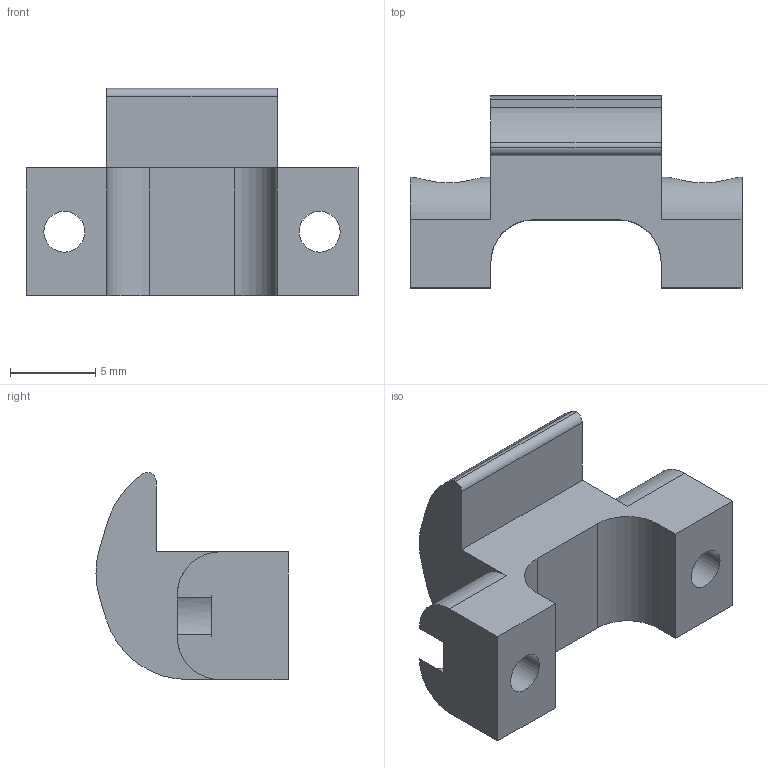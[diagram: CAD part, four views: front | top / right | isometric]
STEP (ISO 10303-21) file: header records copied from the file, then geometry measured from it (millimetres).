
FILE_DESCRIPTION (( 'STEP AP203' ), '1' );
FILE_NAME ('Trigger_Guide.STEP', '2013-11-14T05:08:26', ( '' ), ( '' ), 'SwSTEP 2.0', 'SolidWorks 2013', '' );
FILE_SCHEMA (( 'CONFIG_CONTROL_DESIGN' ));
Length unit declared in the file: millimetre
Products named in the file (1): Trigger_Guide
Bounding box: 19.5 x 11.28 x 12.17 mm (x, y, z)
Volume: 927.9 mm3; surface area: 905.4 mm2
Topology: 1 solids, 1 shells, 42 faces, 117 edges, 77 vertices
Faces by surface type: plane 24, cylinder 18
Entity records: 1511 total; most frequent: CARTESIAN_POINT 313, DIRECTION 240, ORIENTED_EDGE 234, EDGE_CURVE 117, AXIS2_PLACEMENT_3D 84, VERTEX_POINT 77, VECTOR 72, LINE 72
